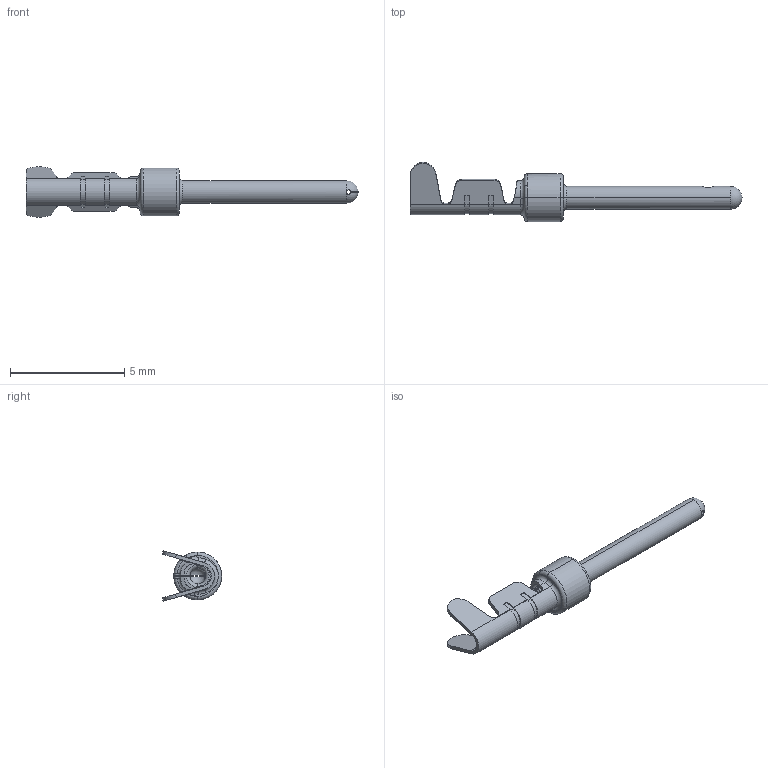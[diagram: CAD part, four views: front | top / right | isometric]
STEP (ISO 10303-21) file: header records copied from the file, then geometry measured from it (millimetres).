
FILE_DESCRIPTION (( 'STEP AP214' ), '1' );
FILE_NAME ('627-290-001.STEP', '2020-09-18T15:59:01', ( '' ), ( '' ), 'SwSTEP 2.0', 'SolidWorks 2020', '' );
FILE_SCHEMA (( 'AUTOMOTIVE_DESIGN' ));
Length unit declared in the file: millimetre
Products named in the file (1): 627-290-001
Bounding box: 14.54 x 2.6 x 2.2 mm (x, y, z)
Volume: 7.7 mm3; surface area: 107.5 mm2
Topology: 1 solids, 1 shells, 189 faces, 527 edges, 336 vertices
Faces by surface type: plane 76, cylinder 75, torus 26, bspline 8, sphere 4
Entity records: 6574 total; most frequent: CARTESIAN_POINT 1739, ORIENTED_EDGE 1038, DIRECTION 983, EDGE_CURVE 519, AXIS2_PLACEMENT_3D 358, VERTEX_POINT 332, VECTOR 267, LINE 267
